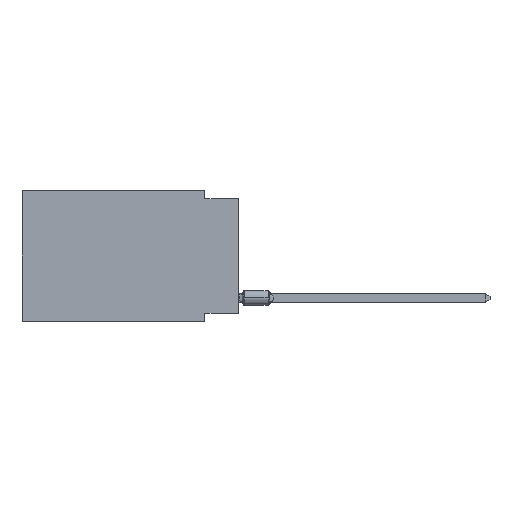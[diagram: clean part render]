
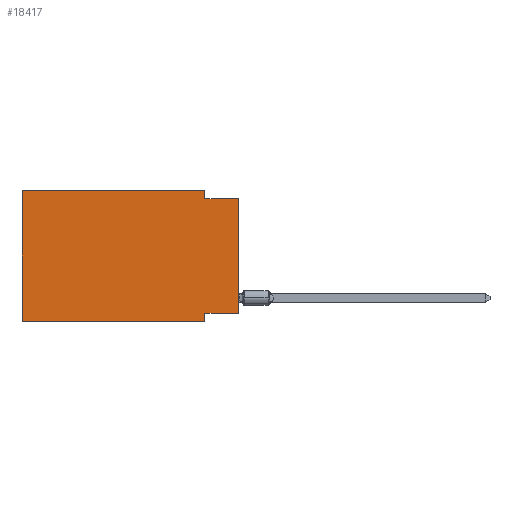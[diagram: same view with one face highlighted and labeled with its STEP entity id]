
A CAD part, left-side view. The second image highlights one B-rep face of the part: STEP entity #18417.
In plain terms, the highlighted planar face has unit normal (-1, 0, 0).
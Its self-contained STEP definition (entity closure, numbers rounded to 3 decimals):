
#219 = EDGE_LOOP ( 'NONE', ( #10387, #30980, #5095, #12154, #25767, #11881, #23536, #19346 ) ) ;
#654 = VECTOR ( 'NONE', #2519, 1000. ) ;
#762 = CARTESIAN_POINT ( 'NONE',  ( 0., 2.54, -0.635 ) ) ;
#1437 = LINE ( 'NONE', #18885, #9932 ) ;
#2335 = CARTESIAN_POINT ( 'NONE',  ( 0., 2.54, 0. ) ) ;
#2358 = CARTESIAN_POINT ( 'NONE',  ( 0., 0., -0.635 ) ) ;
#2388 = EDGE_CURVE ( 'NONE', #22055, #13140, #11837, .T. ) ;
#2503 = DIRECTION ( 'NONE',  ( 0., 0., -1. ) ) ;
#2519 = DIRECTION ( 'NONE',  ( 0., 0., -1. ) ) ;
#3623 = VERTEX_POINT ( 'NONE', #13181 ) ;
#4412 = CARTESIAN_POINT ( 'NONE',  ( 0., 2.54, -9.271 ) ) ;
#4867 = DIRECTION ( 'NONE',  ( 0., 0., 1. ) ) ;
#5095 = ORIENTED_EDGE ( 'NONE', *, *, #18897, .F. ) ;
#6309 = CARTESIAN_POINT ( 'NONE',  ( 0., 16.383, 0. ) ) ;
#7291 = CARTESIAN_POINT ( 'NONE',  ( 0., 16.383, -9.906 ) ) ;
#7472 = VECTOR ( 'NONE', #8066, 1000. ) ;
#7760 = CARTESIAN_POINT ( 'NONE',  ( 0., 16.383, -9.906 ) ) ;
#8066 = DIRECTION ( 'NONE',  ( 0., -1., 0. ) ) ;
#9616 = CARTESIAN_POINT ( 'NONE',  ( 0., 0., -0.635 ) ) ;
#9932 = VECTOR ( 'NONE', #24064, 1000. ) ;
#10371 = VECTOR ( 'NONE', #21369, 1000. ) ;
#10387 = ORIENTED_EDGE ( 'NONE', *, *, #2388, .T. ) ;
#10511 = LINE ( 'NONE', #7760, #7472 ) ;
#10564 = CARTESIAN_POINT ( 'NONE',  ( 0., 16.383, 0. ) ) ;
#11113 = EDGE_CURVE ( 'NONE', #22055, #23794, #1437, .T. ) ;
#11468 = CARTESIAN_POINT ( 'NONE',  ( 0., 2.54, -9.906 ) ) ;
#11608 = EDGE_CURVE ( 'NONE', #23794, #28637, #17230, .T. ) ;
#11726 = LINE ( 'NONE', #9616, #15263 ) ;
#11837 = LINE ( 'NONE', #26891, #24990 ) ;
#11881 = ORIENTED_EDGE ( 'NONE', *, *, #25487, .T. ) ;
#12154 = ORIENTED_EDGE ( 'NONE', *, *, #19975, .F. ) ;
#12653 = VECTOR ( 'NONE', #30873, 1000. ) ;
#13140 = VERTEX_POINT ( 'NONE', #2358 ) ;
#13181 = CARTESIAN_POINT ( 'NONE',  ( 0., 16.383, 0. ) ) ;
#14741 = VERTEX_POINT ( 'NONE', #762 ) ;
#14890 = AXIS2_PLACEMENT_3D ( 'NONE', #10564, #30610, #25448 ) ;
#15033 = VERTEX_POINT ( 'NONE', #23144 ) ;
#15263 = VECTOR ( 'NONE', #29362, 1000. ) ;
#15581 = FACE_OUTER_BOUND ( 'NONE', #219, .T. ) ;
#16311 = LINE ( 'NONE', #21005, #12653 ) ;
#17230 = LINE ( 'NONE', #21914, #654 ) ;
#17474 = VERTEX_POINT ( 'NONE', #7291 ) ;
#18417 = ADVANCED_FACE ( 'NONE', ( #15581 ), #20747, .F. ) ;
#18885 = CARTESIAN_POINT ( 'NONE',  ( 0., 0., -9.271 ) ) ;
#18897 = EDGE_CURVE ( 'NONE', #15033, #14741, #24479, .T. ) ;
#19346 = ORIENTED_EDGE ( 'NONE', *, *, #11113, .F. ) ;
#19975 = EDGE_CURVE ( 'NONE', #3623, #15033, #16311, .T. ) ;
#20747 = PLANE ( 'NONE',  #14890 ) ;
#21005 = CARTESIAN_POINT ( 'NONE',  ( 0., 16.383, 0. ) ) ;
#21369 = DIRECTION ( 'NONE',  ( 0., 0., 1. ) ) ;
#21914 = CARTESIAN_POINT ( 'NONE',  ( 0., 2.54, -9.906 ) ) ;
#22055 = VERTEX_POINT ( 'NONE', #25787 ) ;
#23144 = CARTESIAN_POINT ( 'NONE',  ( 0., 2.54, 0. ) ) ;
#23536 = ORIENTED_EDGE ( 'NONE', *, *, #11608, .F. ) ;
#23794 = VERTEX_POINT ( 'NONE', #4412 ) ;
#24064 = DIRECTION ( 'NONE',  ( 0., 1., 0. ) ) ;
#24128 = EDGE_CURVE ( 'NONE', #17474, #3623, #26057, .T. ) ;
#24479 = LINE ( 'NONE', #2335, #25519 ) ;
#24990 = VECTOR ( 'NONE', #4867, 1000. ) ;
#25448 = DIRECTION ( 'NONE',  ( 0., 0., -1. ) ) ;
#25487 = EDGE_CURVE ( 'NONE', #17474, #28637, #10511, .T. ) ;
#25519 = VECTOR ( 'NONE', #2503, 1000. ) ;
#25767 = ORIENTED_EDGE ( 'NONE', *, *, #24128, .F. ) ;
#25787 = CARTESIAN_POINT ( 'NONE',  ( 0., 0., -9.271 ) ) ;
#26057 = LINE ( 'NONE', #6309, #10371 ) ;
#26891 = CARTESIAN_POINT ( 'NONE',  ( 0., 0., 0. ) ) ;
#27792 = EDGE_CURVE ( 'NONE', #14741, #13140, #11726, .T. ) ;
#28637 = VERTEX_POINT ( 'NONE', #11468 ) ;
#29362 = DIRECTION ( 'NONE',  ( 0., -1., 0. ) ) ;
#30610 = DIRECTION ( 'NONE',  ( 1., 0., 0. ) ) ;
#30873 = DIRECTION ( 'NONE',  ( 0., -1., 0. ) ) ;
#30980 = ORIENTED_EDGE ( 'NONE', *, *, #27792, .F. ) ;
